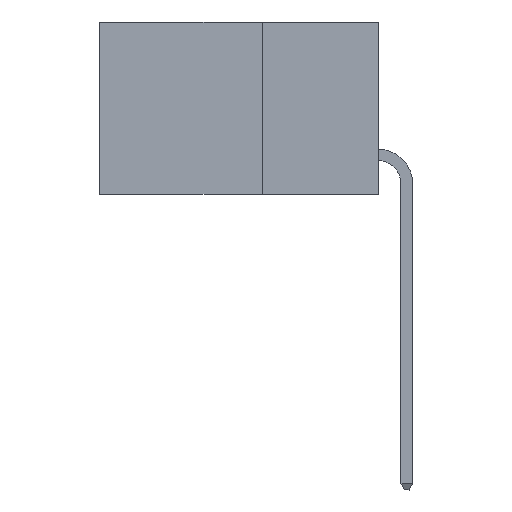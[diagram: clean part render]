
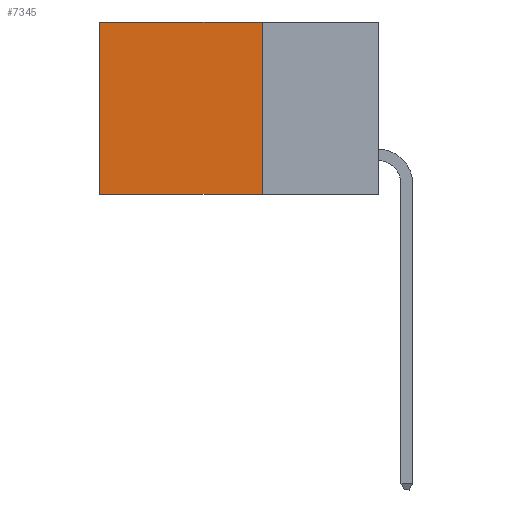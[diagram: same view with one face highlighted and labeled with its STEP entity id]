
A CAD part, left-side view. The second image highlights one B-rep face of the part: STEP entity #7345.
In plain terms, the highlighted planar face has unit normal (-1, 0, 0).
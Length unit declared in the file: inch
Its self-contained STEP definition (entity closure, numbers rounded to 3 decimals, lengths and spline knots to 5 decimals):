
#268 = CARTESIAN_POINT ( 'NONE',  ( 0.2615, 0.6, -0.37 ) ) ;
#566 = VECTOR ( 'NONE', #14450, 39.37008 ) ;
#569 = CARTESIAN_POINT ( 'NONE',  ( 0.2615, 0.25, 0. ) ) ;
#689 = PLANE ( 'NONE',  #13756 ) ;
#1634 = DIRECTION ( 'NONE',  ( 0., 0., -1. ) ) ;
#1680 = LINE ( 'NONE', #569, #3456 ) ;
#2019 = VECTOR ( 'NONE', #13245, 39.37008 ) ;
#2152 = CARTESIAN_POINT ( 'NONE',  ( 0.2615, 0.6, -0.37 ) ) ;
#2344 = CARTESIAN_POINT ( 'NONE',  ( 0.2615, 0.25, 0. ) ) ;
#2719 = EDGE_LOOP ( 'NONE', ( #7476, #8853, #9001, #12766 ) ) ;
#3456 = VECTOR ( 'NONE', #4221, 39.37008 ) ;
#4096 = LINE ( 'NONE', #9803, #566 ) ;
#4221 = DIRECTION ( 'NONE',  ( 0., 1., 0. ) ) ;
#4479 = VERTEX_POINT ( 'NONE', #2152 ) ;
#6445 = CARTESIAN_POINT ( 'NONE',  ( 0.2615, 0.25, -0.37 ) ) ;
#6672 = LINE ( 'NONE', #13398, #2019 ) ;
#6986 = VERTEX_POINT ( 'NONE', #2344 ) ;
#7345 = ADVANCED_FACE ( 'NONE', ( #7406 ), #689, .F. ) ;
#7406 = FACE_OUTER_BOUND ( 'NONE', #2719, .T. ) ;
#7476 = ORIENTED_EDGE ( 'NONE', *, *, #8929, .T. ) ;
#8005 = VECTOR ( 'NONE', #10468, 39.37008 ) ;
#8221 = EDGE_CURVE ( 'NONE', #6986, #10402, #1680, .T. ) ;
#8853 = ORIENTED_EDGE ( 'NONE', *, *, #11692, .F. ) ;
#8929 = EDGE_CURVE ( 'NONE', #10402, #4479, #10548, .T. ) ;
#9001 = ORIENTED_EDGE ( 'NONE', *, *, #10877, .F. ) ;
#9360 = CARTESIAN_POINT ( 'NONE',  ( 0.2615, 0.6, 0. ) ) ;
#9803 = CARTESIAN_POINT ( 'NONE',  ( 0.2615, 0.25, -0.37 ) ) ;
#10334 = VERTEX_POINT ( 'NONE', #13167 ) ;
#10402 = VERTEX_POINT ( 'NONE', #9360 ) ;
#10468 = DIRECTION ( 'NONE',  ( 0., 0., -1. ) ) ;
#10548 = LINE ( 'NONE', #268, #8005 ) ;
#10877 = EDGE_CURVE ( 'NONE', #6986, #10334, #4096, .T. ) ;
#11692 = EDGE_CURVE ( 'NONE', #10334, #4479, #6672, .T. ) ;
#11963 = DIRECTION ( 'NONE',  ( 1., 0., 0. ) ) ;
#12766 = ORIENTED_EDGE ( 'NONE', *, *, #8221, .T. ) ;
#13167 = CARTESIAN_POINT ( 'NONE',  ( 0.2615, 0.25, -0.37 ) ) ;
#13245 = DIRECTION ( 'NONE',  ( 0., 1., 0. ) ) ;
#13398 = CARTESIAN_POINT ( 'NONE',  ( 0.2615, 0.25, -0.37 ) ) ;
#13756 = AXIS2_PLACEMENT_3D ( 'NONE', #6445, #11963, #1634 ) ;
#14450 = DIRECTION ( 'NONE',  ( 0., 0., -1. ) ) ;
